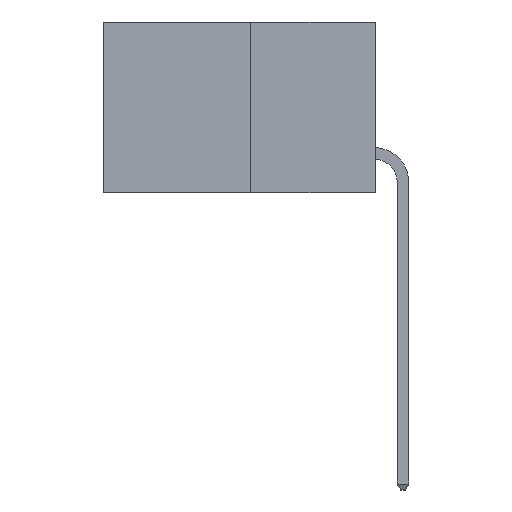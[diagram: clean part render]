
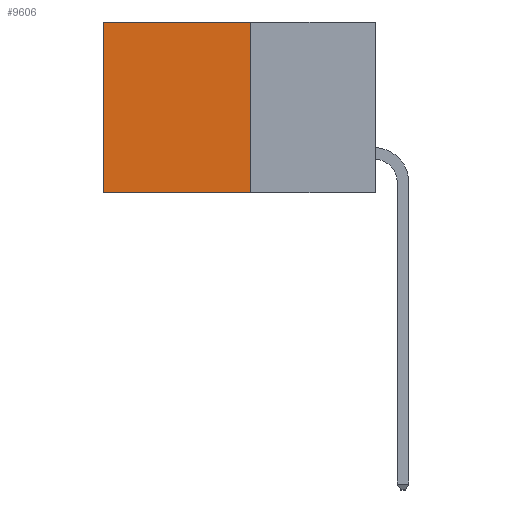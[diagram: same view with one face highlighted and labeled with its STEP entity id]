
A CAD part, left-side view. The second image highlights one B-rep face of the part: STEP entity #9606.
In plain terms, the highlighted planar face has unit normal (-1, 0, 0).
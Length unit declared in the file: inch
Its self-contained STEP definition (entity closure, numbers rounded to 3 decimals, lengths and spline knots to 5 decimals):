
#326 = VECTOR ( 'NONE', #918, 39.37008 ) ;
#918 = DIRECTION ( 'NONE',  ( 0., 0., -1. ) ) ;
#1732 = CARTESIAN_POINT ( 'NONE',  ( 0.277, 0.59, -0.37 ) ) ;
#2081 = VECTOR ( 'NONE', #11966, 39.37008 ) ;
#2530 = EDGE_CURVE ( 'NONE', #14041, #4626, #3848, .T. ) ;
#2856 = ORIENTED_EDGE ( 'NONE', *, *, #4132, .T. ) ;
#2968 = CARTESIAN_POINT ( 'NONE',  ( 0.277, 0.27, 0. ) ) ;
#3010 = VECTOR ( 'NONE', #13078, 39.37008 ) ;
#3848 = LINE ( 'NONE', #7637, #326 ) ;
#4132 = EDGE_CURVE ( 'NONE', #14041, #9672, #16511, .T. ) ;
#4340 = AXIS2_PLACEMENT_3D ( 'NONE', #8046, #7754, #7653 ) ;
#4626 = VERTEX_POINT ( 'NONE', #10460 ) ;
#5635 = LINE ( 'NONE', #10788, #2081 ) ;
#5671 = EDGE_CURVE ( 'NONE', #4626, #8263, #5635, .T. ) ;
#5959 = CARTESIAN_POINT ( 'NONE',  ( 0.277, 0.59, 0. ) ) ;
#6277 = EDGE_LOOP ( 'NONE', ( #6763, #10342, #10902, #2856 ) ) ;
#6483 = DIRECTION ( 'NONE',  ( 0., 0., -1. ) ) ;
#6763 = ORIENTED_EDGE ( 'NONE', *, *, #14324, .T. ) ;
#7182 = CARTESIAN_POINT ( 'NONE',  ( 0.277, 0.27, 0. ) ) ;
#7637 = CARTESIAN_POINT ( 'NONE',  ( 0.277, 0.27, -0.37 ) ) ;
#7653 = DIRECTION ( 'NONE',  ( 0., 0., -1. ) ) ;
#7754 = DIRECTION ( 'NONE',  ( 1., 0., 0. ) ) ;
#8020 = PLANE ( 'NONE',  #4340 ) ;
#8046 = CARTESIAN_POINT ( 'NONE',  ( 0.277, 0.27, -0.37 ) ) ;
#8263 = VERTEX_POINT ( 'NONE', #1732 ) ;
#8895 = VECTOR ( 'NONE', #6483, 39.37008 ) ;
#9088 = CARTESIAN_POINT ( 'NONE',  ( 0.277, 0.59, -0.37 ) ) ;
#9606 = ADVANCED_FACE ( 'NONE', ( #14291 ), #8020, .F. ) ;
#9672 = VERTEX_POINT ( 'NONE', #5959 ) ;
#10342 = ORIENTED_EDGE ( 'NONE', *, *, #5671, .F. ) ;
#10460 = CARTESIAN_POINT ( 'NONE',  ( 0.277, 0.27, -0.37 ) ) ;
#10788 = CARTESIAN_POINT ( 'NONE',  ( 0.277, 0.27, -0.37 ) ) ;
#10902 = ORIENTED_EDGE ( 'NONE', *, *, #2530, .F. ) ;
#11966 = DIRECTION ( 'NONE',  ( 0., 1., 0. ) ) ;
#13078 = DIRECTION ( 'NONE',  ( 0., 1., 0. ) ) ;
#14041 = VERTEX_POINT ( 'NONE', #7182 ) ;
#14291 = FACE_OUTER_BOUND ( 'NONE', #6277, .T. ) ;
#14324 = EDGE_CURVE ( 'NONE', #9672, #8263, #15779, .T. ) ;
#15779 = LINE ( 'NONE', #9088, #8895 ) ;
#16511 = LINE ( 'NONE', #2968, #3010 ) ;
